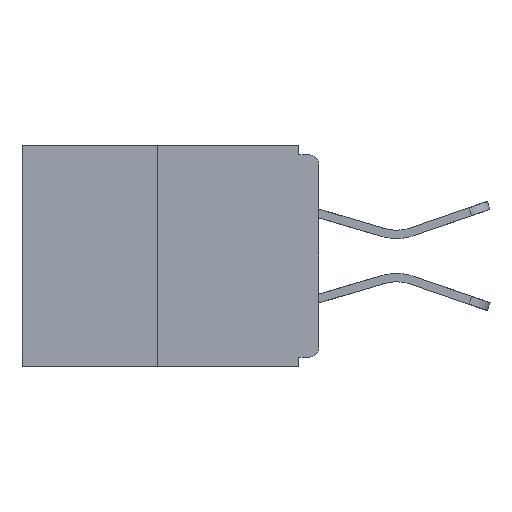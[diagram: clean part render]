
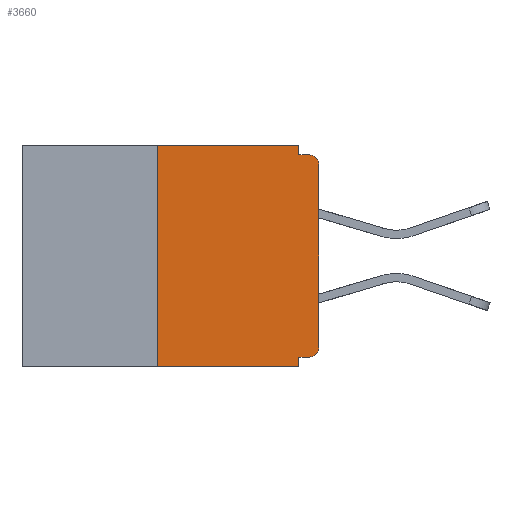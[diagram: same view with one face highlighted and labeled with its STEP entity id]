
A CAD part, left-side view. The second image highlights one B-rep face of the part: STEP entity #3660.
In plain terms, the highlighted planar face has unit normal (-1, 0, 0).
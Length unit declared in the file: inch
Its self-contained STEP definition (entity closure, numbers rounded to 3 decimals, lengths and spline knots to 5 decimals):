
#554 = VERTEX_POINT ( 'NONE', #8952 ) ;
#1514 = DIRECTION ( 'NONE',  ( 0., 0., -1. ) ) ;
#1947 = ORIENTED_EDGE ( 'NONE', *, *, #19806, .T. ) ;
#1953 = VECTOR ( 'NONE', #23657, 39.37008 ) ;
#1982 = LINE ( 'NONE', #7337, #30498 ) ;
#2170 = FACE_OUTER_BOUND ( 'NONE', #3074, .T. ) ;
#2813 = CARTESIAN_POINT ( 'NONE',  ( 0., 0.031, -0.343 ) ) ;
#2836 = EDGE_CURVE ( 'NONE', #6871, #4396, #2860, .T. ) ;
#2860 = LINE ( 'NONE', #25130, #18223 ) ;
#3074 = EDGE_LOOP ( 'NONE', ( #16834, #12442, #12989, #31502, #8233, #7835, #23256, #1947, #25843, #3639 ) ) ;
#3639 = ORIENTED_EDGE ( 'NONE', *, *, #27401, .F. ) ;
#3660 = ADVANCED_FACE ( 'NONE', ( #2170 ), #14197, .F. ) ;
#3696 = EDGE_CURVE ( 'NONE', #4396, #9757, #17618, .T. ) ;
#3848 = DIRECTION ( 'NONE',  ( 0., 0., -1. ) ) ;
#4396 = VERTEX_POINT ( 'NONE', #28417 ) ;
#5865 = AXIS2_PLACEMENT_3D ( 'NONE', #20879, #13873, #1514 ) ;
#6871 = VERTEX_POINT ( 'NONE', #17978 ) ;
#7052 = EDGE_CURVE ( 'NONE', #26055, #20148, #16023, .T. ) ;
#7109 = DIRECTION ( 'NONE',  ( 0., 0., 1. ) ) ;
#7337 = CARTESIAN_POINT ( 'NONE',  ( 0., 0.46, 0. ) ) ;
#7826 = VECTOR ( 'NONE', #7109, 39.37008 ) ;
#7835 = ORIENTED_EDGE ( 'NONE', *, *, #17982, .T. ) ;
#8150 = VECTOR ( 'NONE', #3848, 39.37008 ) ;
#8233 = ORIENTED_EDGE ( 'NONE', *, *, #2836, .F. ) ;
#8391 = EDGE_CURVE ( 'NONE', #30416, #17008, #1982, .T. ) ;
#8805 = CARTESIAN_POINT ( 'NONE',  ( 0., 0.25, 0. ) ) ;
#8952 = CARTESIAN_POINT ( 'NONE',  ( 0., 0.25, -0.343 ) ) ;
#9541 = VERTEX_POINT ( 'NONE', #18542 ) ;
#9545 = CARTESIAN_POINT ( 'NONE',  ( 0., 0., 0. ) ) ;
#9757 = VERTEX_POINT ( 'NONE', #16408 ) ;
#9926 = AXIS2_PLACEMENT_3D ( 'NONE', #22323, #14995, #21838 ) ;
#10505 = DIRECTION ( 'NONE',  ( 0., 1., 0. ) ) ;
#11484 = CIRCLE ( 'NONE', #9926, 0.015 ) ;
#11624 = CARTESIAN_POINT ( 'NONE',  ( 0., 0.46, -0.343 ) ) ;
#11960 = LINE ( 'NONE', #26597, #8150 ) ;
#11991 = LINE ( 'NONE', #24356, #15303 ) ;
#12417 = DIRECTION ( 'NONE',  ( 0., 0., -1. ) ) ;
#12442 = ORIENTED_EDGE ( 'NONE', *, *, #23974, .F. ) ;
#12884 = CARTESIAN_POINT ( 'NONE',  ( 0., 0.015, -0.015 ) ) ;
#12989 = ORIENTED_EDGE ( 'NONE', *, *, #13032, .T. ) ;
#13032 = EDGE_CURVE ( 'NONE', #554, #9757, #31440, .T. ) ;
#13873 = DIRECTION ( 'NONE',  ( -1., 0., 0. ) ) ;
#14197 = PLANE ( 'NONE',  #17504 ) ;
#14490 = VECTOR ( 'NONE', #16046, 39.37008 ) ;
#14995 = DIRECTION ( 'NONE',  ( -1., 0., 0. ) ) ;
#15130 = EDGE_CURVE ( 'NONE', #9541, #26365, #31802, .T. ) ;
#15303 = VECTOR ( 'NONE', #22244, 39.37008 ) ;
#15726 = CIRCLE ( 'NONE', #5865, 0.015 ) ;
#16023 = LINE ( 'NONE', #28531, #1953 ) ;
#16046 = DIRECTION ( 'NONE',  ( 0., -1., 0. ) ) ;
#16408 = CARTESIAN_POINT ( 'NONE',  ( 0., 0.031, -0.343 ) ) ;
#16834 = ORIENTED_EDGE ( 'NONE', *, *, #8391, .F. ) ;
#17008 = VERTEX_POINT ( 'NONE', #26410 ) ;
#17504 = AXIS2_PLACEMENT_3D ( 'NONE', #26894, #26721, #26412 ) ;
#17618 = LINE ( 'NONE', #2813, #27894 ) ;
#17638 = CARTESIAN_POINT ( 'NONE',  ( 0., 0., -0.03 ) ) ;
#17978 = CARTESIAN_POINT ( 'NONE',  ( 0., 0.015, -0.328 ) ) ;
#17982 = EDGE_CURVE ( 'NONE', #6871, #9541, #11484, .T. ) ;
#18223 = VECTOR ( 'NONE', #10505, 39.37008 ) ;
#18542 = CARTESIAN_POINT ( 'NONE',  ( 0., 0., -0.313 ) ) ;
#19806 = EDGE_CURVE ( 'NONE', #26365, #20148, #15726, .T. ) ;
#20148 = VERTEX_POINT ( 'NONE', #12884 ) ;
#20879 = CARTESIAN_POINT ( 'NONE',  ( 0., 0.015, -0.03 ) ) ;
#21838 = DIRECTION ( 'NONE',  ( 0., 0., -1. ) ) ;
#22244 = DIRECTION ( 'NONE',  ( 0., 0., 1. ) ) ;
#22323 = CARTESIAN_POINT ( 'NONE',  ( 0., 0.015, -0.313 ) ) ;
#23040 = CARTESIAN_POINT ( 'NONE',  ( 0., 0.031, -0.015 ) ) ;
#23256 = ORIENTED_EDGE ( 'NONE', *, *, #15130, .T. ) ;
#23657 = DIRECTION ( 'NONE',  ( 0., -1., 0. ) ) ;
#23974 = EDGE_CURVE ( 'NONE', #554, #30416, #11991, .T. ) ;
#24356 = CARTESIAN_POINT ( 'NONE',  ( 0., 0.25, 0. ) ) ;
#25130 = CARTESIAN_POINT ( 'NONE',  ( 0., 0., -0.328 ) ) ;
#25843 = ORIENTED_EDGE ( 'NONE', *, *, #7052, .F. ) ;
#26055 = VERTEX_POINT ( 'NONE', #23040 ) ;
#26365 = VERTEX_POINT ( 'NONE', #17638 ) ;
#26410 = CARTESIAN_POINT ( 'NONE',  ( 0., 0.031, 0. ) ) ;
#26412 = DIRECTION ( 'NONE',  ( 0., 0., -1. ) ) ;
#26597 = CARTESIAN_POINT ( 'NONE',  ( 0., 0.031, 0. ) ) ;
#26688 = DIRECTION ( 'NONE',  ( 0., -1., 0. ) ) ;
#26721 = DIRECTION ( 'NONE',  ( 1., 0., 0. ) ) ;
#26894 = CARTESIAN_POINT ( 'NONE',  ( 0., 0.46, 0. ) ) ;
#27401 = EDGE_CURVE ( 'NONE', #17008, #26055, #11960, .T. ) ;
#27894 = VECTOR ( 'NONE', #12417, 39.37008 ) ;
#28417 = CARTESIAN_POINT ( 'NONE',  ( 0., 0.031, -0.328 ) ) ;
#28531 = CARTESIAN_POINT ( 'NONE',  ( 0., 0., -0.015 ) ) ;
#30416 = VERTEX_POINT ( 'NONE', #8805 ) ;
#30498 = VECTOR ( 'NONE', #26688, 39.37008 ) ;
#31440 = LINE ( 'NONE', #11624, #14490 ) ;
#31502 = ORIENTED_EDGE ( 'NONE', *, *, #3696, .F. ) ;
#31802 = LINE ( 'NONE', #9545, #7826 ) ;
